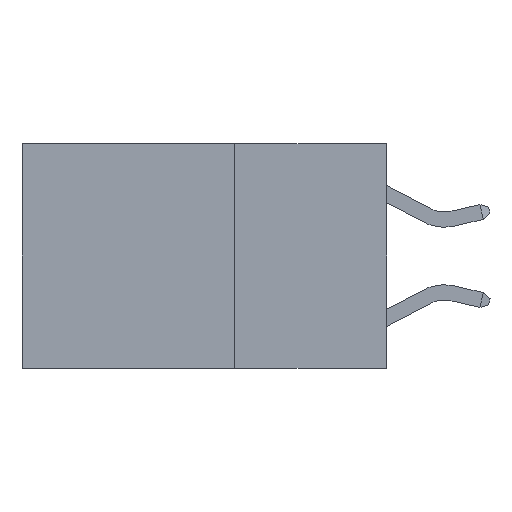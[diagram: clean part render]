
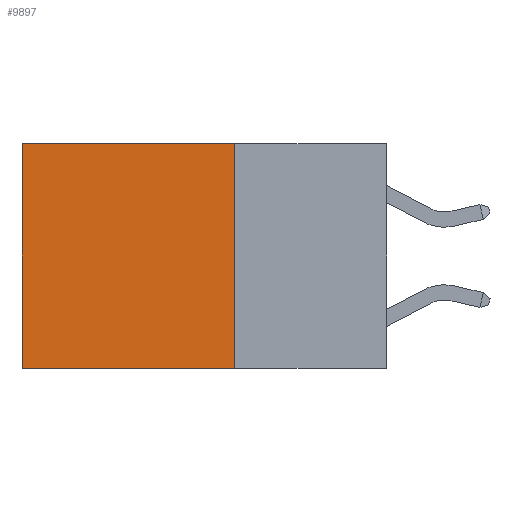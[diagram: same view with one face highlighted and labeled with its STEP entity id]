
A CAD part, left-side view. The second image highlights one B-rep face of the part: STEP entity #9897.
In plain terms, the highlighted planar face has unit normal (-1, 0, 0).
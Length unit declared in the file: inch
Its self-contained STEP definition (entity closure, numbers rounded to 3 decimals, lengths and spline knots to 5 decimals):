
#1758 = CARTESIAN_POINT ( 'NONE',  ( 0.2625, 0.25, 0. ) ) ;
#3187 = VECTOR ( 'NONE', #22316, 39.37008 ) ;
#3874 = DIRECTION ( 'NONE',  ( 0., 0., -1. ) ) ;
#3910 = EDGE_CURVE ( 'NONE', #11798, #16501, #20575, .T. ) ;
#4358 = DIRECTION ( 'NONE',  ( 0., 1., 0. ) ) ;
#5944 = EDGE_LOOP ( 'NONE', ( #18374, #29775, #31547, #16234 ) ) ;
#6894 = EDGE_CURVE ( 'NONE', #21203, #25593, #20352, .T. ) ;
#7532 = CARTESIAN_POINT ( 'NONE',  ( 0.2625, 0.25, -0.37 ) ) ;
#9897 = ADVANCED_FACE ( 'NONE', ( #26265 ), #19054, .F. ) ;
#10519 = EDGE_CURVE ( 'NONE', #16501, #25593, #27486, .T. ) ;
#11798 = VERTEX_POINT ( 'NONE', #27237 ) ;
#13566 = EDGE_CURVE ( 'NONE', #11798, #21203, #24614, .T. ) ;
#15121 = CARTESIAN_POINT ( 'NONE',  ( 0.2625, 0.6, 0. ) ) ;
#15372 = DIRECTION ( 'NONE',  ( 0., 1., 0. ) ) ;
#16059 = VECTOR ( 'NONE', #15372, 39.37008 ) ;
#16234 = ORIENTED_EDGE ( 'NONE', *, *, #13566, .T. ) ;
#16280 = DIRECTION ( 'NONE',  ( 1., 0., 0. ) ) ;
#16501 = VERTEX_POINT ( 'NONE', #26533 ) ;
#16840 = CARTESIAN_POINT ( 'NONE',  ( 0.2625, 0.6, -0.37 ) ) ;
#17882 = CARTESIAN_POINT ( 'NONE',  ( 0.2625, 0.6, 0. ) ) ;
#18111 = DIRECTION ( 'NONE',  ( 0., 0., -1. ) ) ;
#18374 = ORIENTED_EDGE ( 'NONE', *, *, #6894, .T. ) ;
#19054 = PLANE ( 'NONE',  #20073 ) ;
#20073 = AXIS2_PLACEMENT_3D ( 'NONE', #1758, #16280, #3874 ) ;
#20352 = LINE ( 'NONE', #17882, #3187 ) ;
#20575 = LINE ( 'NONE', #30526, #24169 ) ;
#21203 = VERTEX_POINT ( 'NONE', #15121 ) ;
#22316 = DIRECTION ( 'NONE',  ( 0., 0., -1. ) ) ;
#24169 = VECTOR ( 'NONE', #18111, 39.37008 ) ;
#24614 = LINE ( 'NONE', #31954, #29769 ) ;
#25593 = VERTEX_POINT ( 'NONE', #16840 ) ;
#26265 = FACE_OUTER_BOUND ( 'NONE', #5944, .T. ) ;
#26533 = CARTESIAN_POINT ( 'NONE',  ( 0.2625, 0.25, -0.37 ) ) ;
#27237 = CARTESIAN_POINT ( 'NONE',  ( 0.2625, 0.25, 0. ) ) ;
#27486 = LINE ( 'NONE', #7532, #16059 ) ;
#29769 = VECTOR ( 'NONE', #4358, 39.37008 ) ;
#29775 = ORIENTED_EDGE ( 'NONE', *, *, #10519, .F. ) ;
#30526 = CARTESIAN_POINT ( 'NONE',  ( 0.2625, 0.25, 0. ) ) ;
#31547 = ORIENTED_EDGE ( 'NONE', *, *, #3910, .F. ) ;
#31954 = CARTESIAN_POINT ( 'NONE',  ( 0.2625, 0.25, 0. ) ) ;
